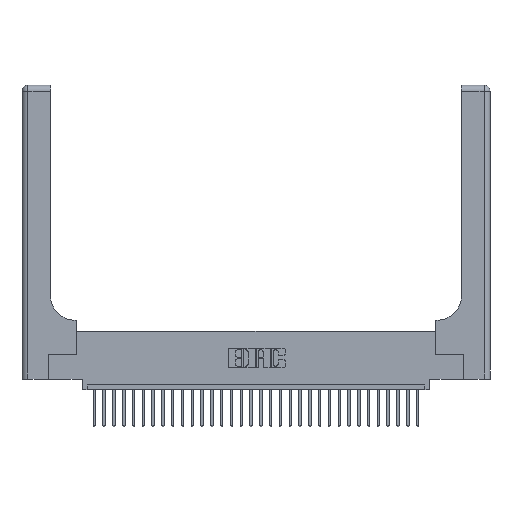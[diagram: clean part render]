
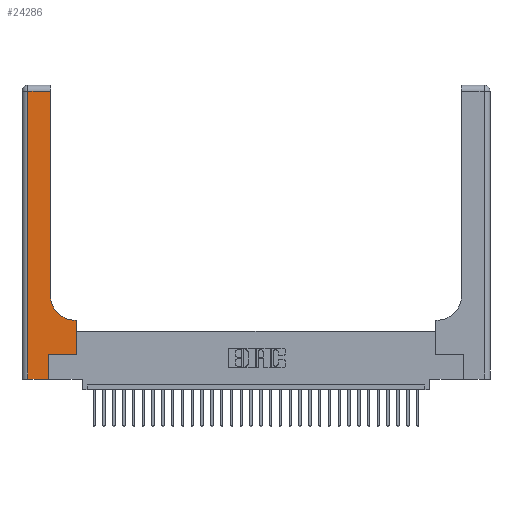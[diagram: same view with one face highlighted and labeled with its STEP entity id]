
A CAD part, top view. The second image highlights one B-rep face of the part: STEP entity #24286.
In plain terms, the highlighted planar face has unit normal (0, 0, 1).
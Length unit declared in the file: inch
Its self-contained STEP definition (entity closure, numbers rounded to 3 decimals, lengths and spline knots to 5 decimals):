
#521 = EDGE_CURVE ( 'NONE', #26858, #1868, #29536, .T. ) ;
#556 = ORIENTED_EDGE ( 'NONE', *, *, #22222, .T. ) ;
#686 = DIRECTION ( 'NONE',  ( 1., 0., 0. ) ) ;
#1568 = CARTESIAN_POINT ( 'NONE',  ( 0., 0., 0.37 ) ) ;
#1705 = VECTOR ( 'NONE', #31468, 39.37008 ) ;
#1868 = VERTEX_POINT ( 'NONE', #31988 ) ;
#2616 = CARTESIAN_POINT ( 'NONE',  ( 0., 3., 0.37 ) ) ;
#4107 = DIRECTION ( 'NONE',  ( 0., 1., 0. ) ) ;
#4794 = CARTESIAN_POINT ( 'NONE',  ( 0.5415, 0.6, 0.37 ) ) ;
#4898 = AXIS2_PLACEMENT_3D ( 'NONE', #6624, #11371, #28648 ) ;
#5083 = CARTESIAN_POINT ( 'NONE',  ( 0.06, 2.94, 0.37 ) ) ;
#5349 = PLANE ( 'NONE',  #31533 ) ;
#5972 = VECTOR ( 'NONE', #18809, 39.37008 ) ;
#6221 = ORIENTED_EDGE ( 'NONE', *, *, #29307, .T. ) ;
#6594 = CIRCLE ( 'NONE', #4898, 0.25 ) ;
#6624 = CARTESIAN_POINT ( 'NONE',  ( 0.5415, 0.85, 0.37 ) ) ;
#6765 = EDGE_CURVE ( 'NONE', #28086, #31230, #6594, .T. ) ;
#6809 = DIRECTION ( 'NONE',  ( 0., -1., 0. ) ) ;
#7374 = EDGE_CURVE ( 'NONE', #23070, #21513, #12732, .T. ) ;
#8756 = CARTESIAN_POINT ( 'NONE',  ( 0.269, 0., 0.37 ) ) ;
#9693 = VECTOR ( 'NONE', #6809, 39.37008 ) ;
#10406 = VECTOR ( 'NONE', #4107, 39.37008 ) ;
#10452 = LINE ( 'NONE', #19197, #9693 ) ;
#10762 = EDGE_LOOP ( 'NONE', ( #6221, #16525, #14756, #28312, #14769, #556, #14282, #20688, #16845 ) ) ;
#11371 = DIRECTION ( 'NONE',  ( 0., 0., -1. ) ) ;
#11631 = LINE ( 'NONE', #11693, #13198 ) ;
#11693 = CARTESIAN_POINT ( 'NONE',  ( 0.2915, 3., 0.37 ) ) ;
#12200 = CARTESIAN_POINT ( 'NONE',  ( 0.5585, 0.25, 0.37 ) ) ;
#12732 = LINE ( 'NONE', #24265, #10406 ) ;
#13135 = CARTESIAN_POINT ( 'NONE',  ( 0.06, 0., 0.37 ) ) ;
#13198 = VECTOR ( 'NONE', #14261, 39.37008 ) ;
#14184 = VECTOR ( 'NONE', #20215, 39.37008 ) ;
#14261 = DIRECTION ( 'NONE',  ( 0., 1., 0. ) ) ;
#14282 = ORIENTED_EDGE ( 'NONE', *, *, #521, .T. ) ;
#14660 = VECTOR ( 'NONE', #23629, 39.37008 ) ;
#14756 = ORIENTED_EDGE ( 'NONE', *, *, #29815, .T. ) ;
#14769 = ORIENTED_EDGE ( 'NONE', *, *, #7374, .T. ) ;
#15447 = CARTESIAN_POINT ( 'NONE',  ( 0.269, 0.25, 0.37 ) ) ;
#16525 = ORIENTED_EDGE ( 'NONE', *, *, #25987, .T. ) ;
#16845 = ORIENTED_EDGE ( 'NONE', *, *, #6765, .T. ) ;
#18809 = DIRECTION ( 'NONE',  ( 1., 0., 0. ) ) ;
#19154 = LINE ( 'NONE', #15447, #25780 ) ;
#19197 = CARTESIAN_POINT ( 'NONE',  ( 0.06, 3., 0.37 ) ) ;
#20116 = VERTEX_POINT ( 'NONE', #5083 ) ;
#20215 = DIRECTION ( 'NONE',  ( -1., 0., 0. ) ) ;
#20688 = ORIENTED_EDGE ( 'NONE', *, *, #30216, .T. ) ;
#21138 = LINE ( 'NONE', #27251, #14184 ) ;
#21513 = VERTEX_POINT ( 'NONE', #27072 ) ;
#21527 = CARTESIAN_POINT ( 'NONE',  ( 0.5585, 0.25, 0.37 ) ) ;
#21609 = LINE ( 'NONE', #26147, #14660 ) ;
#22222 = EDGE_CURVE ( 'NONE', #21513, #26858, #19154, .T. ) ;
#22608 = DIRECTION ( 'NONE',  ( 0., 0., -1. ) ) ;
#23070 = VERTEX_POINT ( 'NONE', #8756 ) ;
#23629 = DIRECTION ( 'NONE',  ( -1., 0., 0. ) ) ;
#24265 = CARTESIAN_POINT ( 'NONE',  ( 0.269, 0., 0.37 ) ) ;
#24286 = ADVANCED_FACE ( 'NONE', ( #28314 ), #5349, .F. ) ;
#24512 = LINE ( 'NONE', #1568, #5972 ) ;
#25780 = VECTOR ( 'NONE', #686, 39.37008 ) ;
#25987 = EDGE_CURVE ( 'NONE', #29390, #20116, #21138, .T. ) ;
#26147 = CARTESIAN_POINT ( 'NONE',  ( 0.2915, 0.6, 0.37 ) ) ;
#26858 = VERTEX_POINT ( 'NONE', #12200 ) ;
#26918 = CARTESIAN_POINT ( 'NONE',  ( 0.2915, 2.94, 0.37 ) ) ;
#27072 = CARTESIAN_POINT ( 'NONE',  ( 0.269, 0.25, 0.37 ) ) ;
#27251 = CARTESIAN_POINT ( 'NONE',  ( 0., 2.94, 0.37 ) ) ;
#27586 = DIRECTION ( 'NONE',  ( -1., 0., 0. ) ) ;
#27780 = VERTEX_POINT ( 'NONE', #13135 ) ;
#27920 = EDGE_CURVE ( 'NONE', #27780, #23070, #24512, .T. ) ;
#28086 = VERTEX_POINT ( 'NONE', #4794 ) ;
#28312 = ORIENTED_EDGE ( 'NONE', *, *, #27920, .T. ) ;
#28314 = FACE_OUTER_BOUND ( 'NONE', #10762, .T. ) ;
#28648 = DIRECTION ( 'NONE',  ( 1., 0., 0. ) ) ;
#29307 = EDGE_CURVE ( 'NONE', #31230, #29390, #11631, .T. ) ;
#29390 = VERTEX_POINT ( 'NONE', #26918 ) ;
#29410 = CARTESIAN_POINT ( 'NONE',  ( 0.2915, 0.85, 0.37 ) ) ;
#29536 = LINE ( 'NONE', #21527, #1705 ) ;
#29815 = EDGE_CURVE ( 'NONE', #20116, #27780, #10452, .T. ) ;
#30216 = EDGE_CURVE ( 'NONE', #1868, #28086, #21609, .T. ) ;
#31230 = VERTEX_POINT ( 'NONE', #29410 ) ;
#31468 = DIRECTION ( 'NONE',  ( 0., 1., 0. ) ) ;
#31533 = AXIS2_PLACEMENT_3D ( 'NONE', #2616, #22608, #27586 ) ;
#31988 = CARTESIAN_POINT ( 'NONE',  ( 0.5585, 0.6, 0.37 ) ) ;
